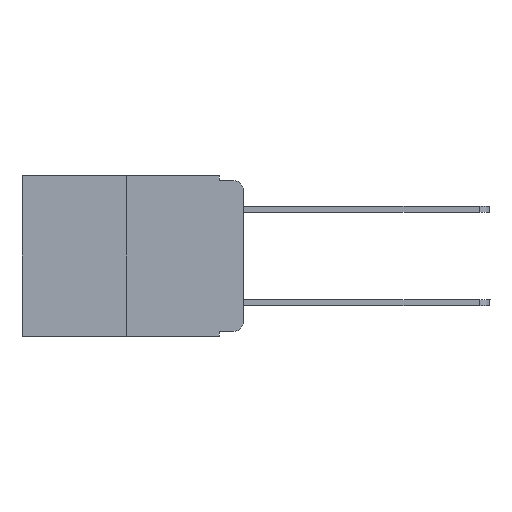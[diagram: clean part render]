
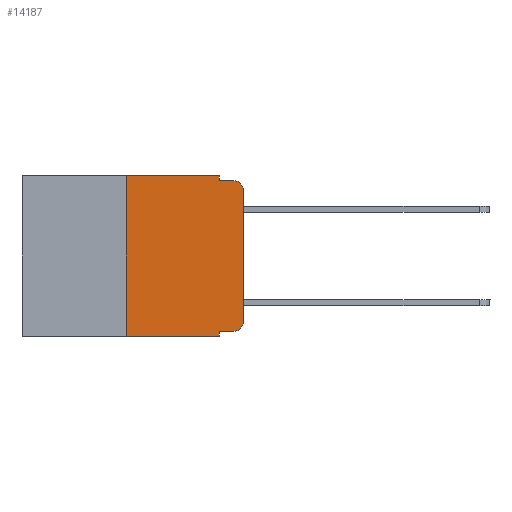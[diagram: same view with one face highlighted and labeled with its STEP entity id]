
A CAD part, left-side view. The second image highlights one B-rep face of the part: STEP entity #14187.
In plain terms, the highlighted planar face has unit normal (-1, 0, 0).
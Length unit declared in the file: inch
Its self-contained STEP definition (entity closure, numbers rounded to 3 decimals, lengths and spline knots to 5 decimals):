
#115 = DIRECTION ( 'NONE',  ( 0., 0., 1. ) ) ;
#571 = DIRECTION ( 'NONE',  ( 0., -1., 0. ) ) ;
#659 = EDGE_CURVE ( 'NONE', #9463, #7085, #12258, .T. ) ;
#706 = VERTEX_POINT ( 'NONE', #9890 ) ;
#732 = CARTESIAN_POINT ( 'NONE',  ( 0., 0.25, 0. ) ) ;
#1378 = DIRECTION ( 'NONE',  ( 0., 0., -1. ) ) ;
#1494 = DIRECTION ( 'NONE',  ( 0., 0., -1. ) ) ;
#1630 = ORIENTED_EDGE ( 'NONE', *, *, #13665, .F. ) ;
#1998 = DIRECTION ( 'NONE',  ( 0., 0., -1. ) ) ;
#2365 = VERTEX_POINT ( 'NONE', #6153 ) ;
#2534 = CARTESIAN_POINT ( 'NONE',  ( 0., 0.02, -0.313 ) ) ;
#2794 = CARTESIAN_POINT ( 'NONE',  ( 0., 0.051, -0.333 ) ) ;
#2819 = CARTESIAN_POINT ( 'NONE',  ( 0., 0.473, 0. ) ) ;
#2868 = EDGE_CURVE ( 'NONE', #2365, #9463, #12788, .T. ) ;
#3023 = CARTESIAN_POINT ( 'NONE',  ( 0., 0.473, 0. ) ) ;
#3207 = VECTOR ( 'NONE', #12820, 39.37008 ) ;
#3292 = CARTESIAN_POINT ( 'NONE',  ( 0., 0.051, -0.333 ) ) ;
#3494 = CIRCLE ( 'NONE', #4709, 0.02 ) ;
#3795 = VECTOR ( 'NONE', #10547, 39.37008 ) ;
#3957 = CARTESIAN_POINT ( 'NONE',  ( 0., 0.051, -0.01 ) ) ;
#4510 = LINE ( 'NONE', #3292, #6151 ) ;
#4664 = VERTEX_POINT ( 'NONE', #2794 ) ;
#4709 = AXIS2_PLACEMENT_3D ( 'NONE', #4838, #14076, #4912 ) ;
#4804 = AXIS2_PLACEMENT_3D ( 'NONE', #2534, #11855, #1378 ) ;
#4838 = CARTESIAN_POINT ( 'NONE',  ( 0., 0.02, -0.03 ) ) ;
#4912 = DIRECTION ( 'NONE',  ( 0., 0., -1. ) ) ;
#5011 = VECTOR ( 'NONE', #13571, 39.37008 ) ;
#5030 = VECTOR ( 'NONE', #1998, 39.37008 ) ;
#5192 = EDGE_CURVE ( 'NONE', #12292, #10281, #8201, .T. ) ;
#5425 = ORIENTED_EDGE ( 'NONE', *, *, #5192, .T. ) ;
#5468 = LINE ( 'NONE', #14717, #5011 ) ;
#6023 = ORIENTED_EDGE ( 'NONE', *, *, #6152, .F. ) ;
#6040 = EDGE_CURVE ( 'NONE', #2365, #706, #8299, .T. ) ;
#6151 = VECTOR ( 'NONE', #7944, 39.37008 ) ;
#6152 = EDGE_CURVE ( 'NONE', #4664, #706, #9105, .T. ) ;
#6153 = CARTESIAN_POINT ( 'NONE',  ( 0., 0.25, -0.343 ) ) ;
#7008 = EDGE_CURVE ( 'NONE', #9370, #14302, #3494, .T. ) ;
#7085 = VERTEX_POINT ( 'NONE', #13313 ) ;
#7554 = CARTESIAN_POINT ( 'NONE',  ( 0., 0.02, -0.01 ) ) ;
#7944 = DIRECTION ( 'NONE',  ( 0., -1., 0. ) ) ;
#8168 = VECTOR ( 'NONE', #11725, 39.37008 ) ;
#8201 = CIRCLE ( 'NONE', #4804, 0.02 ) ;
#8299 = LINE ( 'NONE', #12953, #8168 ) ;
#8883 = ORIENTED_EDGE ( 'NONE', *, *, #12782, .T. ) ;
#9105 = LINE ( 'NONE', #11245, #5030 ) ;
#9370 = VERTEX_POINT ( 'NONE', #13429 ) ;
#9463 = VERTEX_POINT ( 'NONE', #732 ) ;
#9533 = CARTESIAN_POINT ( 'NONE',  ( 0., 0.051, 0. ) ) ;
#9626 = VECTOR ( 'NONE', #571, 39.37008 ) ;
#9654 = LINE ( 'NONE', #11877, #3795 ) ;
#9890 = CARTESIAN_POINT ( 'NONE',  ( 0., 0.051, -0.343 ) ) ;
#9950 = ORIENTED_EDGE ( 'NONE', *, *, #6040, .T. ) ;
#10137 = EDGE_LOOP ( 'NONE', ( #8883, #14555, #11840, #1630, #10609, #10567, #9950, #6023, #12026, #5425 ) ) ;
#10197 = CARTESIAN_POINT ( 'NONE',  ( 0., 0., -0.313 ) ) ;
#10281 = VERTEX_POINT ( 'NONE', #10197 ) ;
#10547 = DIRECTION ( 'NONE',  ( 0., 0., 1. ) ) ;
#10567 = ORIENTED_EDGE ( 'NONE', *, *, #2868, .F. ) ;
#10609 = ORIENTED_EDGE ( 'NONE', *, *, #659, .F. ) ;
#11064 = VERTEX_POINT ( 'NONE', #3957 ) ;
#11245 = CARTESIAN_POINT ( 'NONE',  ( 0., 0.051, 0. ) ) ;
#11363 = CARTESIAN_POINT ( 'NONE',  ( 0., 0.02, -0.333 ) ) ;
#11725 = DIRECTION ( 'NONE',  ( 0., -1., 0. ) ) ;
#11840 = ORIENTED_EDGE ( 'NONE', *, *, #14340, .F. ) ;
#11855 = DIRECTION ( 'NONE',  ( -1., 0., 0. ) ) ;
#11877 = CARTESIAN_POINT ( 'NONE',  ( 0., 0., 0. ) ) ;
#11968 = FACE_OUTER_BOUND ( 'NONE', #10137, .T. ) ;
#12026 = ORIENTED_EDGE ( 'NONE', *, *, #13481, .T. ) ;
#12194 = PLANE ( 'NONE',  #12534 ) ;
#12258 = LINE ( 'NONE', #3023, #9626 ) ;
#12292 = VERTEX_POINT ( 'NONE', #11363 ) ;
#12534 = AXIS2_PLACEMENT_3D ( 'NONE', #2819, #13116, #1494 ) ;
#12782 = EDGE_CURVE ( 'NONE', #10281, #9370, #9654, .T. ) ;
#12788 = LINE ( 'NONE', #13024, #15117 ) ;
#12820 = DIRECTION ( 'NONE',  ( 0., 0., -1. ) ) ;
#12953 = CARTESIAN_POINT ( 'NONE',  ( 0., 0.473, -0.343 ) ) ;
#13024 = CARTESIAN_POINT ( 'NONE',  ( 0., 0.25, 0. ) ) ;
#13116 = DIRECTION ( 'NONE',  ( 1., 0., 0. ) ) ;
#13313 = CARTESIAN_POINT ( 'NONE',  ( 0., 0.051, 0. ) ) ;
#13429 = CARTESIAN_POINT ( 'NONE',  ( 0., 0., -0.03 ) ) ;
#13481 = EDGE_CURVE ( 'NONE', #4664, #12292, #4510, .T. ) ;
#13571 = DIRECTION ( 'NONE',  ( 0., -1., 0. ) ) ;
#13665 = EDGE_CURVE ( 'NONE', #7085, #11064, #13968, .T. ) ;
#13968 = LINE ( 'NONE', #9533, #3207 ) ;
#14076 = DIRECTION ( 'NONE',  ( -1., 0., 0. ) ) ;
#14187 = ADVANCED_FACE ( 'NONE', ( #11968 ), #12194, .F. ) ;
#14302 = VERTEX_POINT ( 'NONE', #7554 ) ;
#14340 = EDGE_CURVE ( 'NONE', #11064, #14302, #5468, .T. ) ;
#14555 = ORIENTED_EDGE ( 'NONE', *, *, #7008, .T. ) ;
#14717 = CARTESIAN_POINT ( 'NONE',  ( 0., 0.051, -0.01 ) ) ;
#15117 = VECTOR ( 'NONE', #115, 39.37008 ) ;
